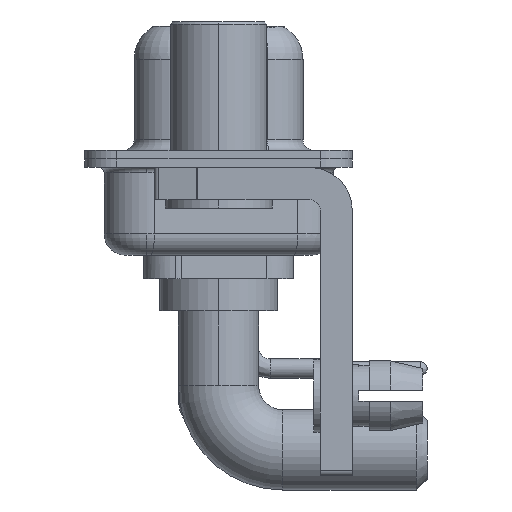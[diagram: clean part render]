
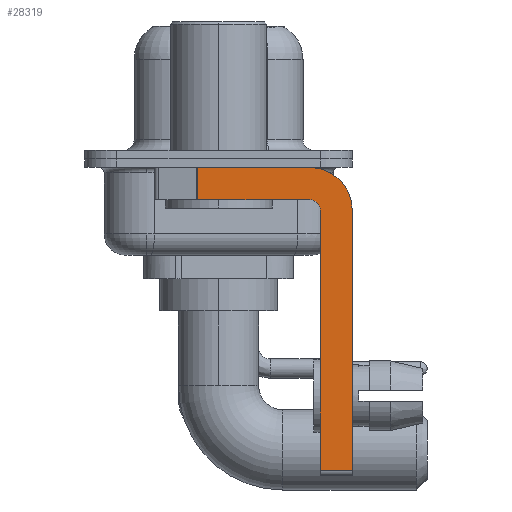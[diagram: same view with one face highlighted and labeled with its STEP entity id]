
A CAD part, left-side view. The second image highlights one B-rep face of the part: STEP entity #28319.
In plain terms, the highlighted planar face has unit normal (-1, 0, 0).
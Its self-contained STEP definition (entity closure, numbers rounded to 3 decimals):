
#305 = VERTEX_POINT ( 'NONE', #16441 ) ;
#427 = DIRECTION ( 'NONE',  ( 1., 0., 0. ) ) ;
#635 = CARTESIAN_POINT ( 'NONE',  ( -2.9, -4.25, -1.9 ) ) ;
#1117 = VERTEX_POINT ( 'NONE', #9195 ) ;
#1756 = CARTESIAN_POINT ( 'NONE',  ( -2.9, 3., -0.4 ) ) ;
#2812 = CIRCLE ( 'NONE', #17028, 0.5 ) ;
#2886 = CARTESIAN_POINT ( 'NONE',  ( -2.9, -4.25, -2.4 ) ) ;
#3046 = VERTEX_POINT ( 'NONE', #15322 ) ;
#3608 = ORIENTED_EDGE ( 'NONE', *, *, #16503, .F. ) ;
#3756 = VECTOR ( 'NONE', #11192, 1000. ) ;
#4575 = ORIENTED_EDGE ( 'NONE', *, *, #8024, .F. ) ;
#4664 = EDGE_CURVE ( 'NONE', #13793, #3046, #17113, .T. ) ;
#5221 = DIRECTION ( 'NONE',  ( 1., 0., 0. ) ) ;
#5468 = ORIENTED_EDGE ( 'NONE', *, *, #13377, .T. ) ;
#5793 = ORIENTED_EDGE ( 'NONE', *, *, #17508, .F. ) ;
#5930 = DIRECTION ( 'NONE',  ( 0., -1., 0. ) ) ;
#6394 = CIRCLE ( 'NONE', #25638, 2. ) ;
#7317 = DIRECTION ( 'NONE',  ( 0., 0., 1. ) ) ;
#7464 = DIRECTION ( 'NONE',  ( 0., 1., 0. ) ) ;
#7658 = FACE_OUTER_BOUND ( 'NONE', #20509, .T. ) ;
#7959 = VERTEX_POINT ( 'NONE', #28321 ) ;
#8024 = EDGE_CURVE ( 'NONE', #7959, #28368, #2812, .T. ) ;
#8610 = CARTESIAN_POINT ( 'NONE',  ( -2.9, -4.25, -2.4 ) ) ;
#8663 = DIRECTION ( 'NONE',  ( -1., 0., 0. ) ) ;
#9195 = CARTESIAN_POINT ( 'NONE',  ( -2.9, -6.25, -2.4 ) ) ;
#9372 = ORIENTED_EDGE ( 'NONE', *, *, #4664, .F. ) ;
#9532 = CARTESIAN_POINT ( 'NONE',  ( -2.9, -6.25, -2.4 ) ) ;
#11053 = LINE ( 'NONE', #11331, #3756 ) ;
#11113 = EDGE_CURVE ( 'NONE', #28368, #24135, #16521, .T. ) ;
#11145 = VECTOR ( 'NONE', #11268, 1000. ) ;
#11192 = DIRECTION ( 'NONE',  ( 0., 0., -1. ) ) ;
#11268 = DIRECTION ( 'NONE',  ( 0., 0., -1. ) ) ;
#11331 = CARTESIAN_POINT ( 'NONE',  ( -2.9, 0.978, -1.9 ) ) ;
#11434 = EDGE_CURVE ( 'NONE', #3046, #1117, #6394, .T. ) ;
#11784 = AXIS2_PLACEMENT_3D ( 'NONE', #14259, #5221, #26765 ) ;
#12342 = CARTESIAN_POINT ( 'NONE',  ( -2.9, -4.25, -14.55 ) ) ;
#13233 = DIRECTION ( 'NONE',  ( 0., 0., 1. ) ) ;
#13377 = EDGE_CURVE ( 'NONE', #13793, #24135, #11053, .T. ) ;
#13625 = CARTESIAN_POINT ( 'NONE',  ( -2.9, -4.25, -1.9 ) ) ;
#13679 = LINE ( 'NONE', #9532, #11145 ) ;
#13793 = VERTEX_POINT ( 'NONE', #17305 ) ;
#14113 = PLANE ( 'NONE',  #11784 ) ;
#14153 = VECTOR ( 'NONE', #7464, 1000. ) ;
#14259 = CARTESIAN_POINT ( 'NONE',  ( -2.9, -4.25, -2.4 ) ) ;
#14397 = VECTOR ( 'NONE', #7317, 1000. ) ;
#15322 = CARTESIAN_POINT ( 'NONE',  ( -2.9, -4.25, -0.4 ) ) ;
#15358 = CARTESIAN_POINT ( 'NONE',  ( -2.9, 0.978, -1.9 ) ) ;
#16238 = DIRECTION ( 'NONE',  ( 0., -1., 0. ) ) ;
#16441 = CARTESIAN_POINT ( 'NONE',  ( -2.9, -6.25, -14.55 ) ) ;
#16503 = EDGE_CURVE ( 'NONE', #1117, #305, #13679, .T. ) ;
#16521 = LINE ( 'NONE', #13625, #14153 ) ;
#17028 = AXIS2_PLACEMENT_3D ( 'NONE', #2886, #8663, #13233 ) ;
#17113 = LINE ( 'NONE', #1756, #19245 ) ;
#17305 = CARTESIAN_POINT ( 'NONE',  ( -2.9, 0.978, -0.4 ) ) ;
#17504 = DIRECTION ( 'NONE',  ( 0., 0., -1. ) ) ;
#17508 = EDGE_CURVE ( 'NONE', #26680, #7959, #26986, .T. ) ;
#18677 = CARTESIAN_POINT ( 'NONE',  ( -2.9, -4.75, -14.8 ) ) ;
#19227 = ORIENTED_EDGE ( 'NONE', *, *, #11113, .F. ) ;
#19245 = VECTOR ( 'NONE', #5930, 1000. ) ;
#20509 = EDGE_LOOP ( 'NONE', ( #9372, #5468, #19227, #4575, #5793, #23960, #3608, #27856 ) ) ;
#20961 = LINE ( 'NONE', #12342, #23193 ) ;
#23168 = CARTESIAN_POINT ( 'NONE',  ( -2.9, -4.75, -14.55 ) ) ;
#23193 = VECTOR ( 'NONE', #16238, 1000. ) ;
#23960 = ORIENTED_EDGE ( 'NONE', *, *, #27101, .T. ) ;
#24135 = VERTEX_POINT ( 'NONE', #15358 ) ;
#25638 = AXIS2_PLACEMENT_3D ( 'NONE', #8610, #427, #17504 ) ;
#26680 = VERTEX_POINT ( 'NONE', #23168 ) ;
#26765 = DIRECTION ( 'NONE',  ( 0., 0., -1. ) ) ;
#26986 = LINE ( 'NONE', #18677, #14397 ) ;
#27101 = EDGE_CURVE ( 'NONE', #26680, #305, #20961, .T. ) ;
#27856 = ORIENTED_EDGE ( 'NONE', *, *, #11434, .F. ) ;
#28319 = ADVANCED_FACE ( 'NONE', ( #7658 ), #14113, .F. ) ;
#28321 = CARTESIAN_POINT ( 'NONE',  ( -2.9, -4.75, -2.4 ) ) ;
#28368 = VERTEX_POINT ( 'NONE', #635 ) ;
